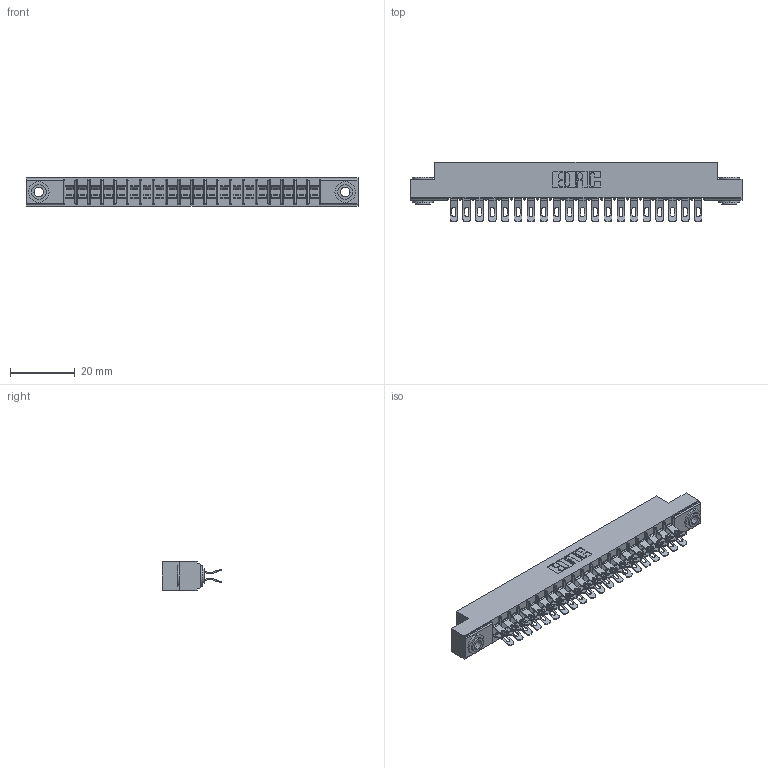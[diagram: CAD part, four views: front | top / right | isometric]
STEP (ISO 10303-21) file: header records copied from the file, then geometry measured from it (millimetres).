
FILE_DESCRIPTION (( 'STEP AP203' ), '1' );
FILE_NAME ('315-040-555-203.STEP', '2019-09-10T17:22:05', ( '' ), ( '' ), 'SwSTEP 2.0', 'SolidWorks 2016', '' );
FILE_SCHEMA (( 'CONFIG_CONTROL_DESIGN' ));
Length unit declared in the file: inch
Products named in the file (4): 305-290-001_555; 345-250-002_345-250-002-102; 305 Part_.156 Dia; 315-040-555-203
Assembly tree (43 placements, depth 2):
  315-040-555-203
    305 Part_.156 Dia
    305-290-001_555  x40
    345-250-002_345-250-002-102  x2
Bounding box: 102.26 x 18.41 x 8.71 mm (x, y, z)
Volume: 6539.9 mm3; surface area: 13146.7 mm2
Topology: 43 solids, 43 shells, 2808 faces, 8328 edges, 5440 vertices
Faces by surface type: plane 1372, cylinder 1348, sphere 80, cone 8
Entity records: 26022 total; most frequent: CARTESIAN_POINT 4305, ORIENTED_EDGE 4252, DIRECTION 4192, EDGE_CURVE 2126, VECTOR 1666, LINE 1666, VERTEX_POINT 1360, AXIS2_PLACEMENT_3D 1263
